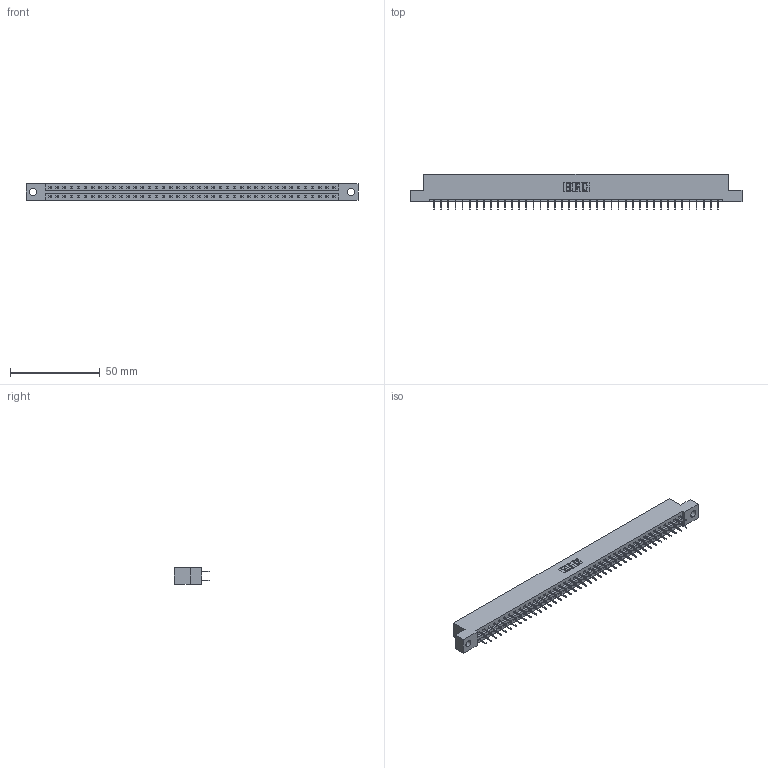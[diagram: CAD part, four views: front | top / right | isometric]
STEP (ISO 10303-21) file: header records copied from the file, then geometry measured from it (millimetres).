
FILE_DESCRIPTION (( 'STEP AP203' ), '1' );
FILE_NAME ('337-082-524-204.STEP', '2019-10-10T12:57:56', ( '' ), ( '' ), 'SwSTEP 2.0', 'SolidWorks 2016', '' );
FILE_SCHEMA (( 'CONFIG_CONTROL_DESIGN' ));
Length unit declared in the file: inch
Products named in the file (3): 345-292-001_345-293-124; 337 Part_Flush Mounting Lugs - 0.156 Dia-TH; 337-082-524-204
Assembly tree (83 placements, depth 2):
  337-082-524-204
    337 Part_Flush Mounting Lugs - 0.156 Dia-TH
    345-292-001_345-293-124  x82
Bounding box: 185.47 x 19.69 x 9.4 mm (x, y, z)
Volume: 19321.1 mm3; surface area: 21245.9 mm2
Topology: 83 solids, 83 shells, 4870 faces, 13841 edges, 8898 vertices
Faces by surface type: plane 3678, cylinder 1192
Entity records: 31995 total; most frequent: CARTESIAN_POINT 5390, ORIENTED_EDGE 5326, DIRECTION 4587, EDGE_CURVE 2663, VECTOR 2539, LINE 2539, VERTEX_POINT 1770, AXIS2_PLACEMENT_3D 1024
